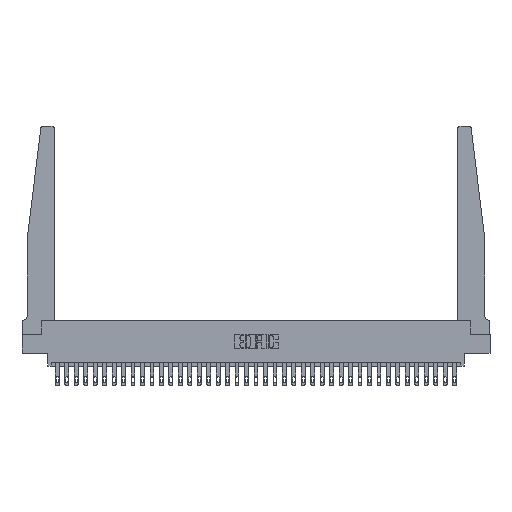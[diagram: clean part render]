
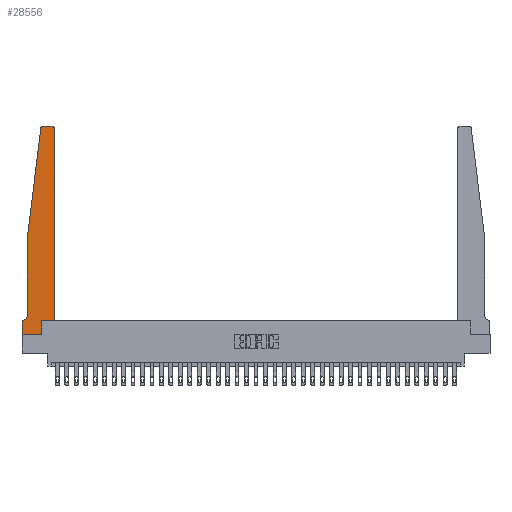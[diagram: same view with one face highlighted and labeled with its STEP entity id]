
A CAD part, top view. The second image highlights one B-rep face of the part: STEP entity #28556.
In plain terms, the highlighted planar face has unit normal (0, 0, 1).
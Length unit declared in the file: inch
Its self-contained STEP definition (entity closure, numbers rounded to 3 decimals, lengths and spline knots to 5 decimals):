
#15 = VERTEX_POINT ( 'NONE', #22012 ) ;
#150 = CARTESIAN_POINT ( 'NONE',  ( 0.2605, 0., 0.37 ) ) ;
#425 = VERTEX_POINT ( 'NONE', #26468 ) ;
#634 = CARTESIAN_POINT ( 'NONE',  ( 0.425, 0.18, 0.37 ) ) ;
#798 = VERTEX_POINT ( 'NONE', #26756 ) ;
#1027 = DIRECTION ( 'NONE',  ( -1., 0., 0. ) ) ;
#1248 = ORIENTED_EDGE ( 'NONE', *, *, #22780, .T. ) ;
#1282 = CARTESIAN_POINT ( 'NONE',  ( 0.425, 0.18, 0.37 ) ) ;
#1311 = AXIS2_PLACEMENT_3D ( 'NONE', #30995, #30835, #7798 ) ;
#1326 = CARTESIAN_POINT ( 'NONE',  ( 0.015, 0.1875, 0.37 ) ) ;
#1908 = CARTESIAN_POINT ( 'NONE',  ( 0., 0., 0.37 ) ) ;
#1930 = DIRECTION ( 'NONE',  ( 0., 0., 1. ) ) ;
#2159 = EDGE_CURVE ( 'NONE', #11309, #6402, #29231, .T. ) ;
#3759 = CARTESIAN_POINT ( 'NONE',  ( 0.24675, 2.72367, 0.37 ) ) ;
#4256 = CARTESIAN_POINT ( 'NONE',  ( 0.27653, 2.75, 0.37 ) ) ;
#4414 = AXIS2_PLACEMENT_3D ( 'NONE', #24178, #23687, #10886 ) ;
#4934 = LINE ( 'NONE', #1908, #16921 ) ;
#5231 = EDGE_CURVE ( 'NONE', #6402, #7052, #20305, .T. ) ;
#5459 = DIRECTION ( 'NONE',  ( 1., 0., 0. ) ) ;
#6402 = VERTEX_POINT ( 'NONE', #18921 ) ;
#6948 = DIRECTION ( 'NONE',  ( 0., 0., 1. ) ) ;
#7052 = VERTEX_POINT ( 'NONE', #27723 ) ;
#7194 = VECTOR ( 'NONE', #28904, 39.37008 ) ;
#7705 = EDGE_CURVE ( 'NONE', #15, #11309, #15423, .T. ) ;
#7798 = DIRECTION ( 'NONE',  ( 1., 0., 0. ) ) ;
#7952 = EDGE_CURVE ( 'NONE', #28208, #15505, #24087, .T. ) ;
#8156 = VECTOR ( 'NONE', #25290, 39.37008 ) ;
#8468 = EDGE_LOOP ( 'NONE', ( #30701, #20589, #14419, #1248, #28301, #8658, #17508, #27458, #23791, #17281, #22650, #32107 ) ) ;
#8658 = ORIENTED_EDGE ( 'NONE', *, *, #18739, .T. ) ;
#8785 = CARTESIAN_POINT ( 'NONE',  ( 0., 0.1875, 0.37 ) ) ;
#9559 = AXIS2_PLACEMENT_3D ( 'NONE', #14880, #6948, #25299 ) ;
#9686 = EDGE_CURVE ( 'NONE', #7052, #28208, #11300, .T. ) ;
#10340 = LINE ( 'NONE', #31172, #20520 ) ;
#10651 = VERTEX_POINT ( 'NONE', #8785 ) ;
#10662 = FACE_OUTER_BOUND ( 'NONE', #8468, .T. ) ;
#10734 = VECTOR ( 'NONE', #1027, 39.37008 ) ;
#10886 = DIRECTION ( 'NONE',  ( -1., 0., 0. ) ) ;
#11300 = LINE ( 'NONE', #29299, #10734 ) ;
#11309 = VERTEX_POINT ( 'NONE', #634 ) ;
#11596 = VECTOR ( 'NONE', #18672, 39.37008 ) ;
#12360 = DIRECTION ( 'NONE',  ( 1., 0., 0. ) ) ;
#12403 = LINE ( 'NONE', #19667, #13214 ) ;
#12724 = VERTEX_POINT ( 'NONE', #150 ) ;
#13214 = VECTOR ( 'NONE', #17805, 39.37008 ) ;
#13984 = EDGE_CURVE ( 'NONE', #15505, #425, #25456, .T. ) ;
#14419 = ORIENTED_EDGE ( 'NONE', *, *, #13984, .T. ) ;
#14880 = CARTESIAN_POINT ( 'NONE',  ( 0.27653, 2.72, 0.37 ) ) ;
#15250 = CARTESIAN_POINT ( 'NONE',  ( 0.425, 0.18, 0.37 ) ) ;
#15423 = LINE ( 'NONE', #15250, #23568 ) ;
#15505 = VERTEX_POINT ( 'NONE', #3759 ) ;
#16921 = VECTOR ( 'NONE', #17907, 39.37008 ) ;
#17281 = ORIENTED_EDGE ( 'NONE', *, *, #7705, .T. ) ;
#17282 = VECTOR ( 'NONE', #30810, 39.37008 ) ;
#17508 = ORIENTED_EDGE ( 'NONE', *, *, #28416, .T. ) ;
#17646 = VERTEX_POINT ( 'NONE', #1326 ) ;
#17805 = DIRECTION ( 'NONE',  ( -1., 0., 0. ) ) ;
#17865 = CIRCLE ( 'NONE', #4414, 0.05 ) ;
#17907 = DIRECTION ( 'NONE',  ( 0., -1., 0. ) ) ;
#18672 = DIRECTION ( 'NONE',  ( 0., 1., 0. ) ) ;
#18739 = EDGE_CURVE ( 'NONE', #17646, #10651, #12403, .T. ) ;
#18921 = CARTESIAN_POINT ( 'NONE',  ( 0.425, 2.72, 0.37 ) ) ;
#19667 = CARTESIAN_POINT ( 'NONE',  ( 0.065, 0.1875, 0.37 ) ) ;
#20252 = LINE ( 'NONE', #32985, #8156 ) ;
#20305 = CIRCLE ( 'NONE', #24060, 0.03 ) ;
#20520 = VECTOR ( 'NONE', #28159, 39.37008 ) ;
#20589 = ORIENTED_EDGE ( 'NONE', *, *, #7952, .T. ) ;
#21043 = LINE ( 'NONE', #31421, #11596 ) ;
#22012 = CARTESIAN_POINT ( 'NONE',  ( 0.2605, 0.18, 0.37 ) ) ;
#22650 = ORIENTED_EDGE ( 'NONE', *, *, #2159, .T. ) ;
#22780 = EDGE_CURVE ( 'NONE', #425, #798, #20252, .T. ) ;
#22937 = CARTESIAN_POINT ( 'NONE',  ( 0.065, 1.25, 0.37 ) ) ;
#22957 = EDGE_CURVE ( 'NONE', #30055, #12724, #10340, .T. ) ;
#23286 = PLANE ( 'NONE',  #1311 ) ;
#23568 = VECTOR ( 'NONE', #5459, 39.37008 ) ;
#23687 = DIRECTION ( 'NONE',  ( 0., 0., -1. ) ) ;
#23791 = ORIENTED_EDGE ( 'NONE', *, *, #30591, .T. ) ;
#24060 = AXIS2_PLACEMENT_3D ( 'NONE', #29868, #1930, #12360 ) ;
#24087 = CIRCLE ( 'NONE', #9559, 0.03 ) ;
#24178 = CARTESIAN_POINT ( 'NONE',  ( 0.015, 0.2375, 0.37 ) ) ;
#25290 = DIRECTION ( 'NONE',  ( 0., -1., 0. ) ) ;
#25299 = DIRECTION ( 'NONE',  ( 1., 0., 0. ) ) ;
#25456 = LINE ( 'NONE', #22937, #17282 ) ;
#25792 = EDGE_CURVE ( 'NONE', #798, #17646, #17865, .T. ) ;
#26468 = CARTESIAN_POINT ( 'NONE',  ( 0.065, 1.25, 0.37 ) ) ;
#26756 = CARTESIAN_POINT ( 'NONE',  ( 0.065, 0.2375, 0.37 ) ) ;
#27458 = ORIENTED_EDGE ( 'NONE', *, *, #22957, .T. ) ;
#27723 = CARTESIAN_POINT ( 'NONE',  ( 0.395, 2.75, 0.37 ) ) ;
#28159 = DIRECTION ( 'NONE',  ( 1., 0., 0. ) ) ;
#28208 = VERTEX_POINT ( 'NONE', #4256 ) ;
#28287 = CARTESIAN_POINT ( 'NONE',  ( 0., 0., 0.37 ) ) ;
#28301 = ORIENTED_EDGE ( 'NONE', *, *, #25792, .T. ) ;
#28416 = EDGE_CURVE ( 'NONE', #10651, #30055, #4934, .T. ) ;
#28556 = ADVANCED_FACE ( 'NONE', ( #10662 ), #23286, .T. ) ;
#28904 = DIRECTION ( 'NONE',  ( 0., 1., 0. ) ) ;
#29231 = LINE ( 'NONE', #1282, #7194 ) ;
#29299 = CARTESIAN_POINT ( 'NONE',  ( 0.25, 2.75, 0.37 ) ) ;
#29868 = CARTESIAN_POINT ( 'NONE',  ( 0.395, 2.72, 0.37 ) ) ;
#30055 = VERTEX_POINT ( 'NONE', #28287 ) ;
#30591 = EDGE_CURVE ( 'NONE', #12724, #15, #21043, .T. ) ;
#30701 = ORIENTED_EDGE ( 'NONE', *, *, #9686, .T. ) ;
#30810 = DIRECTION ( 'NONE',  ( -0.122, -0.992, 0. ) ) ;
#30835 = DIRECTION ( 'NONE',  ( 0., 0., 1. ) ) ;
#30995 = CARTESIAN_POINT ( 'NONE',  ( 0., 0.1875, 0.37 ) ) ;
#31172 = CARTESIAN_POINT ( 'NONE',  ( 0., 0., 0.37 ) ) ;
#31421 = CARTESIAN_POINT ( 'NONE',  ( 0.2605, 0.18, 0.37 ) ) ;
#32107 = ORIENTED_EDGE ( 'NONE', *, *, #5231, .T. ) ;
#32985 = CARTESIAN_POINT ( 'NONE',  ( 0.065, 1.25, 0.37 ) ) ;
